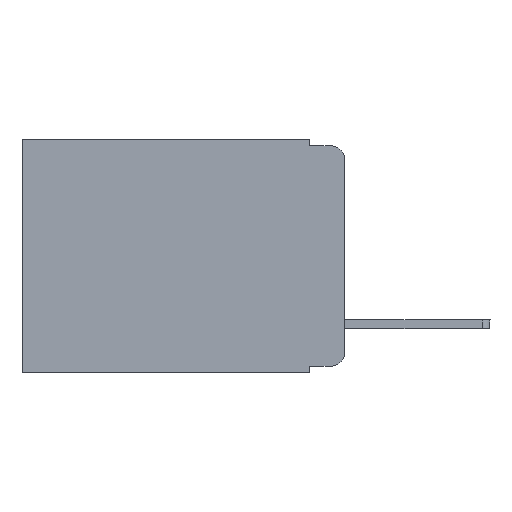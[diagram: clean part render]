
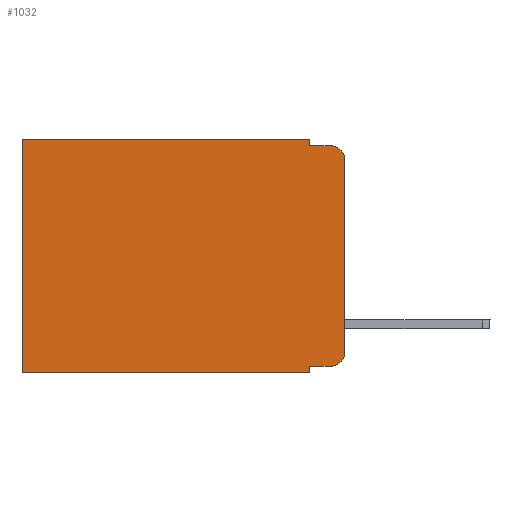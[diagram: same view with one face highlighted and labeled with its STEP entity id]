
A CAD part, left-side view. The second image highlights one B-rep face of the part: STEP entity #1032.
In plain terms, the highlighted planar face has unit normal (-1, 0, 0).
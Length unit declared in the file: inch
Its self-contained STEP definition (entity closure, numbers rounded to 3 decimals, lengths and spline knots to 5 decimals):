
#25 = CARTESIAN_POINT ( 'NONE',  ( 0.298, 0., -0.313 ) ) ;
#352 = LINE ( 'NONE', #2666, #16942 ) ;
#562 = CARTESIAN_POINT ( 'NONE',  ( 0.298, 0.473, 0. ) ) ;
#1032 = ADVANCED_FACE ( 'NONE', ( #7774 ), #12002, .F. ) ;
#1093 = CARTESIAN_POINT ( 'NONE',  ( 0.298, 0.051, -0.343 ) ) ;
#1440 = CIRCLE ( 'NONE', #4587, 0.02 ) ;
#1960 = ORIENTED_EDGE ( 'NONE', *, *, #9383, .F. ) ;
#2098 = CARTESIAN_POINT ( 'NONE',  ( 0.298, 0., 0. ) ) ;
#2194 = EDGE_CURVE ( 'NONE', #9609, #9319, #7723, .T. ) ;
#2433 = DIRECTION ( 'NONE',  ( 0., 0., -1. ) ) ;
#2666 = CARTESIAN_POINT ( 'NONE',  ( 0.298, 0., 0. ) ) ;
#2681 = CARTESIAN_POINT ( 'NONE',  ( 0.298, 0.051, -0.333 ) ) ;
#2825 = VERTEX_POINT ( 'NONE', #6423 ) ;
#3077 = ORIENTED_EDGE ( 'NONE', *, *, #15385, .T. ) ;
#3874 = DIRECTION ( 'NONE',  ( 0., 0., -1. ) ) ;
#4274 = LINE ( 'NONE', #15853, #17783 ) ;
#4290 = ORIENTED_EDGE ( 'NONE', *, *, #9455, .F. ) ;
#4326 = DIRECTION ( 'NONE',  ( 0., -1., 0. ) ) ;
#4348 = CARTESIAN_POINT ( 'NONE',  ( 0.298, 0.473, -0.343 ) ) ;
#4587 = AXIS2_PLACEMENT_3D ( 'NONE', #13689, #17840, #12197 ) ;
#4667 = CIRCLE ( 'NONE', #11865, 0.02 ) ;
#5115 = DIRECTION ( 'NONE',  ( -1., 0., 0. ) ) ;
#5164 = DIRECTION ( 'NONE',  ( 0., 0., -1. ) ) ;
#5262 = EDGE_CURVE ( 'NONE', #10462, #16729, #7391, .T. ) ;
#5852 = CARTESIAN_POINT ( 'NONE',  ( 0.298, 0.051, -0.333 ) ) ;
#6274 = ORIENTED_EDGE ( 'NONE', *, *, #6641, .F. ) ;
#6370 = LINE ( 'NONE', #13428, #9014 ) ;
#6423 = CARTESIAN_POINT ( 'NONE',  ( 0.298, 0.02, -0.01 ) ) ;
#6641 = EDGE_CURVE ( 'NONE', #9778, #8269, #11707, .T. ) ;
#6980 = DIRECTION ( 'NONE',  ( 0., -1., 0. ) ) ;
#7050 = CARTESIAN_POINT ( 'NONE',  ( 0.298, 0.051, -0.01 ) ) ;
#7324 = ORIENTED_EDGE ( 'NONE', *, *, #5262, .F. ) ;
#7391 = LINE ( 'NONE', #9341, #12401 ) ;
#7410 = EDGE_CURVE ( 'NONE', #9319, #15935, #4667, .T. ) ;
#7723 = LINE ( 'NONE', #2681, #9251 ) ;
#7726 = VERTEX_POINT ( 'NONE', #562 ) ;
#7774 = FACE_OUTER_BOUND ( 'NONE', #17338, .T. ) ;
#8269 = VERTEX_POINT ( 'NONE', #4348 ) ;
#8325 = VECTOR ( 'NONE', #6980, 39.37008 ) ;
#8399 = ORIENTED_EDGE ( 'NONE', *, *, #7410, .T. ) ;
#8450 = DIRECTION ( 'NONE',  ( 0., 0., -1. ) ) ;
#8537 = VECTOR ( 'NONE', #8450, 39.37008 ) ;
#8753 = LINE ( 'NONE', #7050, #8325 ) ;
#9014 = VECTOR ( 'NONE', #14845, 39.37008 ) ;
#9251 = VECTOR ( 'NONE', #4326, 39.37008 ) ;
#9319 = VERTEX_POINT ( 'NONE', #10749 ) ;
#9341 = CARTESIAN_POINT ( 'NONE',  ( 0.298, 0.051, 0. ) ) ;
#9383 = EDGE_CURVE ( 'NONE', #9609, #9778, #9401, .T. ) ;
#9401 = LINE ( 'NONE', #12646, #8537 ) ;
#9455 = EDGE_CURVE ( 'NONE', #16729, #2825, #8753, .T. ) ;
#9609 = VERTEX_POINT ( 'NONE', #5852 ) ;
#9778 = VERTEX_POINT ( 'NONE', #1093 ) ;
#10049 = CARTESIAN_POINT ( 'NONE',  ( 0.298, 0., -0.03 ) ) ;
#10205 = CARTESIAN_POINT ( 'NONE',  ( 0.298, 0.051, -0.01 ) ) ;
#10462 = VERTEX_POINT ( 'NONE', #17894 ) ;
#10749 = CARTESIAN_POINT ( 'NONE',  ( 0.298, 0.02, -0.333 ) ) ;
#11288 = CARTESIAN_POINT ( 'NONE',  ( 0.298, 0., -0.343 ) ) ;
#11707 = LINE ( 'NONE', #11288, #17785 ) ;
#11784 = EDGE_CURVE ( 'NONE', #10462, #7726, #352, .T. ) ;
#11865 = AXIS2_PLACEMENT_3D ( 'NONE', #17835, #5115, #3874 ) ;
#11936 = DIRECTION ( 'NONE',  ( 1., 0., 0. ) ) ;
#12002 = PLANE ( 'NONE',  #14204 ) ;
#12139 = VERTEX_POINT ( 'NONE', #10049 ) ;
#12197 = DIRECTION ( 'NONE',  ( 0., 0., -1. ) ) ;
#12401 = VECTOR ( 'NONE', #2433, 39.37008 ) ;
#12646 = CARTESIAN_POINT ( 'NONE',  ( 0.298, 0.051, 0. ) ) ;
#13097 = DIRECTION ( 'NONE',  ( 0., 0., -1. ) ) ;
#13327 = ORIENTED_EDGE ( 'NONE', *, *, #11784, .T. ) ;
#13391 = ORIENTED_EDGE ( 'NONE', *, *, #2194, .T. ) ;
#13428 = CARTESIAN_POINT ( 'NONE',  ( 0.298, 0.473, 0. ) ) ;
#13689 = CARTESIAN_POINT ( 'NONE',  ( 0.298, 0.02, -0.03 ) ) ;
#13710 = EDGE_CURVE ( 'NONE', #12139, #15935, #4274, .T. ) ;
#14151 = ORIENTED_EDGE ( 'NONE', *, *, #15747, .T. ) ;
#14204 = AXIS2_PLACEMENT_3D ( 'NONE', #2098, #11936, #5164 ) ;
#14845 = DIRECTION ( 'NONE',  ( 0., 0., -1. ) ) ;
#15385 = EDGE_CURVE ( 'NONE', #7726, #8269, #6370, .T. ) ;
#15747 = EDGE_CURVE ( 'NONE', #12139, #2825, #1440, .T. ) ;
#15853 = CARTESIAN_POINT ( 'NONE',  ( 0.298, 0., 0. ) ) ;
#15935 = VERTEX_POINT ( 'NONE', #25 ) ;
#16630 = DIRECTION ( 'NONE',  ( 0., 1., 0. ) ) ;
#16706 = DIRECTION ( 'NONE',  ( 0., 1., 0. ) ) ;
#16729 = VERTEX_POINT ( 'NONE', #10205 ) ;
#16806 = ORIENTED_EDGE ( 'NONE', *, *, #13710, .F. ) ;
#16942 = VECTOR ( 'NONE', #16630, 39.37008 ) ;
#17338 = EDGE_LOOP ( 'NONE', ( #16806, #14151, #4290, #7324, #13327, #3077, #6274, #1960, #13391, #8399 ) ) ;
#17783 = VECTOR ( 'NONE', #13097, 39.37008 ) ;
#17785 = VECTOR ( 'NONE', #16706, 39.37008 ) ;
#17835 = CARTESIAN_POINT ( 'NONE',  ( 0.298, 0.02, -0.313 ) ) ;
#17840 = DIRECTION ( 'NONE',  ( -1., 0., 0. ) ) ;
#17894 = CARTESIAN_POINT ( 'NONE',  ( 0.298, 0.051, 0. ) ) ;
